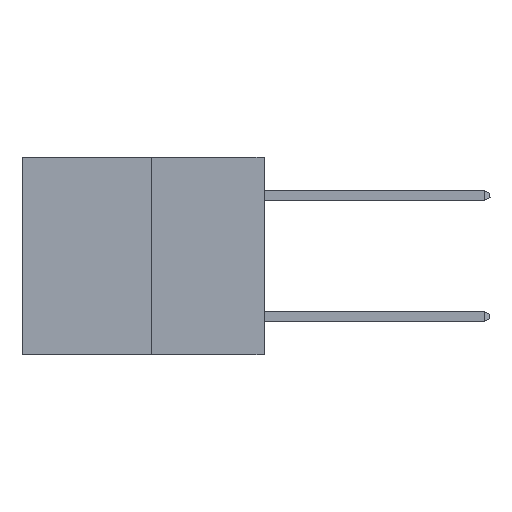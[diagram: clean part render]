
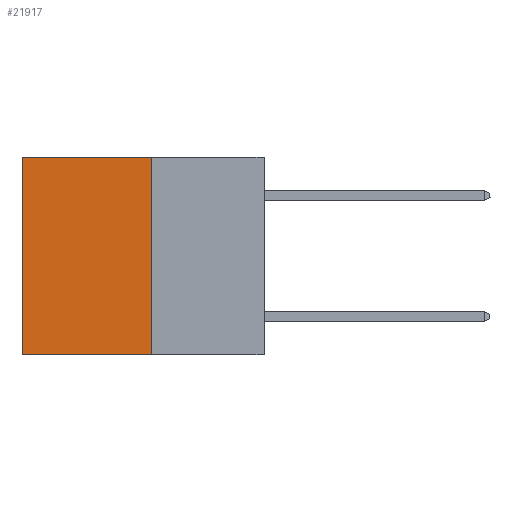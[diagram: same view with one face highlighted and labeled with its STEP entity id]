
A CAD part, left-side view. The second image highlights one B-rep face of the part: STEP entity #21917.
In plain terms, the highlighted planar face has unit normal (-1, 0, 0).
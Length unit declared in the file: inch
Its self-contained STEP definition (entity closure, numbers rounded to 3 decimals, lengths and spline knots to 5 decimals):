
#660 = PLANE ( 'NONE',  #15456 ) ;
#1392 = VECTOR ( 'NONE', #15149, 39.37008 ) ;
#1518 = VECTOR ( 'NONE', #21520, 39.37008 ) ;
#2241 = CARTESIAN_POINT ( 'NONE',  ( 0.3165, 0.28, 0. ) ) ;
#2300 = ORIENTED_EDGE ( 'NONE', *, *, #12331, .F. ) ;
#2370 = CARTESIAN_POINT ( 'NONE',  ( 0.3165, 0.6, 0. ) ) ;
#2675 = LINE ( 'NONE', #19456, #1392 ) ;
#2865 = VERTEX_POINT ( 'NONE', #2241 ) ;
#2872 = VERTEX_POINT ( 'NONE', #25002 ) ;
#3453 = DIRECTION ( 'NONE',  ( 0., 0., -1. ) ) ;
#5013 = FACE_OUTER_BOUND ( 'NONE', #19049, .T. ) ;
#5455 = DIRECTION ( 'NONE',  ( 0., 1., 0. ) ) ;
#6094 = ORIENTED_EDGE ( 'NONE', *, *, #7692, .T. ) ;
#6101 = CARTESIAN_POINT ( 'NONE',  ( 0.3165, 0.28, -0.49 ) ) ;
#7692 = EDGE_CURVE ( 'NONE', #2865, #21737, #2675, .T. ) ;
#9067 = LINE ( 'NONE', #18076, #26418 ) ;
#10436 = LINE ( 'NONE', #24220, #20946 ) ;
#12331 = EDGE_CURVE ( 'NONE', #2865, #25865, #23782, .T. ) ;
#12840 = ORIENTED_EDGE ( 'NONE', *, *, #17900, .F. ) ;
#15149 = DIRECTION ( 'NONE',  ( 0., 1., 0. ) ) ;
#15456 = AXIS2_PLACEMENT_3D ( 'NONE', #25980, #15885, #3453 ) ;
#15885 = DIRECTION ( 'NONE',  ( 1., 0., 0. ) ) ;
#17543 = ORIENTED_EDGE ( 'NONE', *, *, #25704, .T. ) ;
#17900 = EDGE_CURVE ( 'NONE', #25865, #2872, #10436, .T. ) ;
#18076 = CARTESIAN_POINT ( 'NONE',  ( 0.3165, 0.6, -0.49 ) ) ;
#19049 = EDGE_LOOP ( 'NONE', ( #17543, #12840, #2300, #6094 ) ) ;
#19456 = CARTESIAN_POINT ( 'NONE',  ( 0.3165, 0.28, 0. ) ) ;
#20946 = VECTOR ( 'NONE', #5455, 39.37008 ) ;
#21520 = DIRECTION ( 'NONE',  ( 0., 0., -1. ) ) ;
#21737 = VERTEX_POINT ( 'NONE', #2370 ) ;
#21917 = ADVANCED_FACE ( 'NONE', ( #5013 ), #660, .F. ) ;
#22587 = CARTESIAN_POINT ( 'NONE',  ( 0.3165, 0.28, -0.49 ) ) ;
#23782 = LINE ( 'NONE', #22587, #1518 ) ;
#23990 = DIRECTION ( 'NONE',  ( 0., 0., -1. ) ) ;
#24220 = CARTESIAN_POINT ( 'NONE',  ( 0.3165, 0.28, -0.49 ) ) ;
#25002 = CARTESIAN_POINT ( 'NONE',  ( 0.3165, 0.6, -0.49 ) ) ;
#25704 = EDGE_CURVE ( 'NONE', #21737, #2872, #9067, .T. ) ;
#25865 = VERTEX_POINT ( 'NONE', #6101 ) ;
#25980 = CARTESIAN_POINT ( 'NONE',  ( 0.3165, 0.28, -0.49 ) ) ;
#26418 = VECTOR ( 'NONE', #23990, 39.37008 ) ;
